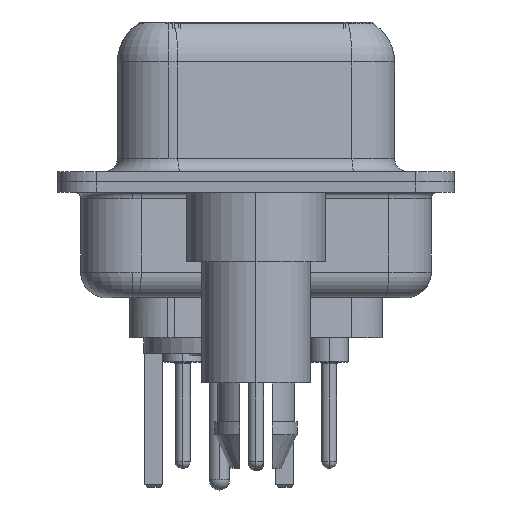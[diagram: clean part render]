
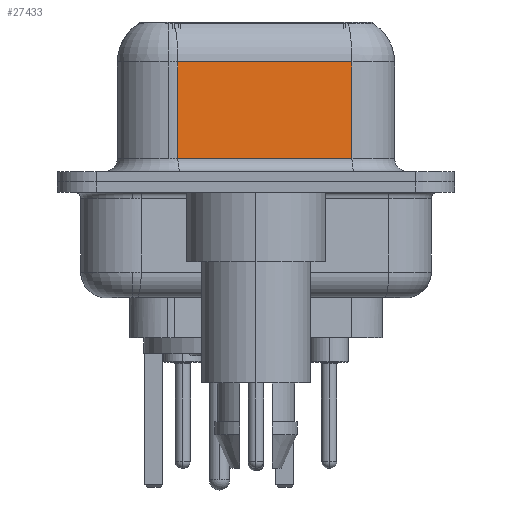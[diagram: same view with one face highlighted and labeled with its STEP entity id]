
A CAD part, left-side view. The second image highlights one B-rep face of the part: STEP entity #27433.
In plain terms, the highlighted planar face has unit normal (-0.985, -0.174, 0).
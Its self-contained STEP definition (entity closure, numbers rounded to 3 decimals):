
#18 = LINE ( 'NONE', #2135, #5900 ) ;
#195 = DIRECTION ( 'NONE',  ( 0.985, 0.174, 0. ) ) ;
#712 = LINE ( 'NONE', #23015, #16706 ) ;
#1762 = ORIENTED_EDGE ( 'NONE', *, *, #26022, .T. ) ;
#2135 = CARTESIAN_POINT ( 'NONE',  ( 5.621, -3.722, 6.4 ) ) ;
#2159 = CARTESIAN_POINT ( 'NONE',  ( 5.621, -3.722, 4.65 ) ) ;
#3268 = ORIENTED_EDGE ( 'NONE', *, *, #11943, .T. ) ;
#3354 = DIRECTION ( 'NONE',  ( 0., 0., -1. ) ) ;
#3601 = VERTEX_POINT ( 'NONE', #2159 ) ;
#3669 = LINE ( 'NONE', #22213, #9972 ) ;
#3798 = CARTESIAN_POINT ( 'NONE',  ( 5.621, -3.722, 0.9 ) ) ;
#4131 = EDGE_CURVE ( 'NONE', #3601, #17460, #18, .T. ) ;
#5900 = VECTOR ( 'NONE', #10815, 1000. ) ;
#6985 = VERTEX_POINT ( 'NONE', #32542 ) ;
#7617 = ORIENTED_EDGE ( 'NONE', *, *, #25889, .T. ) ;
#9972 = VECTOR ( 'NONE', #3354, 1000. ) ;
#10815 = DIRECTION ( 'NONE',  ( 0., 0., -1. ) ) ;
#11943 = EDGE_CURVE ( 'NONE', #3601, #16533, #23558, .T. ) ;
#12730 = ORIENTED_EDGE ( 'NONE', *, *, #4131, .F. ) ;
#15565 = CARTESIAN_POINT ( 'NONE',  ( 4.43, 3.028, 4.65 ) ) ;
#16533 = VERTEX_POINT ( 'NONE', #15565 ) ;
#16547 = PLANE ( 'NONE',  #19152 ) ;
#16706 = VECTOR ( 'NONE', #17826, 1000. ) ;
#17460 = VERTEX_POINT ( 'NONE', #3798 ) ;
#17826 = DIRECTION ( 'NONE',  ( 0.174, -0.985, 0. ) ) ;
#18469 = EDGE_LOOP ( 'NONE', ( #12730, #3268, #7617, #1762 ) ) ;
#19152 = AXIS2_PLACEMENT_3D ( 'NONE', #27036, #195, #29632 ) ;
#22213 = CARTESIAN_POINT ( 'NONE',  ( 4.43, 3.028, 6.4 ) ) ;
#23015 = CARTESIAN_POINT ( 'NONE',  ( 5.621, -3.722, 0.9 ) ) ;
#23558 = LINE ( 'NONE', #32624, #27770 ) ;
#25089 = FACE_OUTER_BOUND ( 'NONE', #18469, .T. ) ;
#25889 = EDGE_CURVE ( 'NONE', #16533, #6985, #3669, .T. ) ;
#26022 = EDGE_CURVE ( 'NONE', #6985, #17460, #712, .T. ) ;
#27036 = CARTESIAN_POINT ( 'NONE',  ( 5.621, -3.722, 6.4 ) ) ;
#27340 = DIRECTION ( 'NONE',  ( -0.174, 0.985, 0. ) ) ;
#27433 = ADVANCED_FACE ( 'NONE', ( #25089 ), #16547, .F. ) ;
#27770 = VECTOR ( 'NONE', #27340, 1000. ) ;
#29632 = DIRECTION ( 'NONE',  ( -0.174, 0.985, 0. ) ) ;
#32542 = CARTESIAN_POINT ( 'NONE',  ( 4.43, 3.028, 0.9 ) ) ;
#32624 = CARTESIAN_POINT ( 'NONE',  ( 5.621, -3.722, 4.65 ) ) ;
